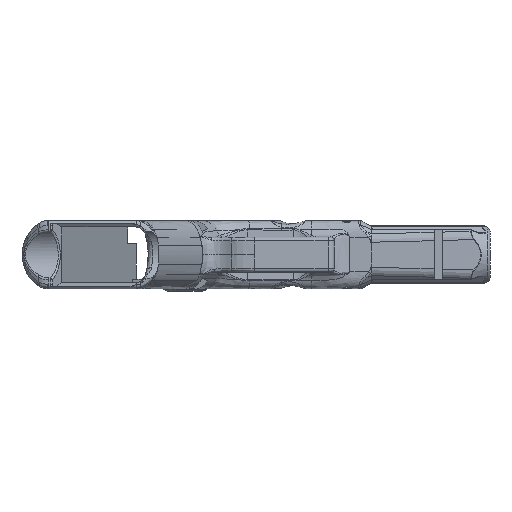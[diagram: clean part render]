
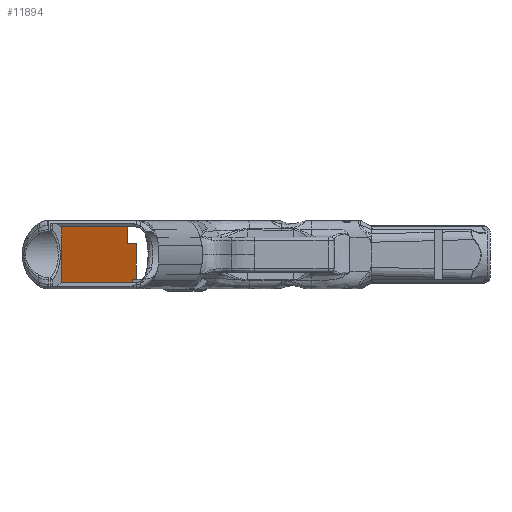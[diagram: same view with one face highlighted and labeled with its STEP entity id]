
A CAD part, front view. The second image highlights one B-rep face of the part: STEP entity #11894.
In plain terms, the highlighted planar face has unit normal (0.951, -0.309, 0).
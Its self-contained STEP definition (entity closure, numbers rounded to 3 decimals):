
#684=ELLIPSE('',#12474,1.051,1.);
#694=ELLIPSE('',#12501,1.051,1.);
#1610=FACE_OUTER_BOUND('',#2282,.T.);
#2282=EDGE_LOOP('',(#10482,#10483,#10484,#10485,#10486,#10487,#10488,#10489,
#10490,#10491));
#3350=LINE('',#25282,#4028);
#3474=LINE('',#29733,#4152);
#3485=LINE('',#30019,#4163);
#3627=LINE('',#42026,#4305);
#3650=LINE('',#43778,#4328);
#3654=LINE('',#44102,#4332);
#3660=LINE('',#44735,#4338);
#3661=LINE('',#44736,#4339);
#4028=VECTOR('',#13857,10.);
#4152=VECTOR('',#14323,10.);
#4163=VECTOR('',#14362,10.);
#4305=VECTOR('',#14990,10.);
#4328=VECTOR('',#15133,10.);
#4332=VECTOR('',#15141,10.);
#4338=VECTOR('',#15177,10.);
#4339=VECTOR('',#15178,10.);
#4899=VERTEX_POINT('',#25279);
#4900=VERTEX_POINT('',#25281);
#5053=VERTEX_POINT('',#28687);
#5094=VERTEX_POINT('',#29708);
#5096=VERTEX_POINT('',#29712);
#5104=VERTEX_POINT('',#29731);
#5458=VERTEX_POINT('',#42024);
#5495=VERTEX_POINT('',#43777);
#5502=VERTEX_POINT('',#44099);
#5503=VERTEX_POINT('',#44101);
#6274=EDGE_CURVE('',#4900,#4899,#3350,.T.);
#6515=EDGE_CURVE('',#5053,#4899,#684,.F.);
#6574=EDGE_CURVE('',#5096,#5094,#694,.F.);
#6584=EDGE_CURVE('',#5096,#5104,#3474,.T.);
#6614=EDGE_CURVE('',#5094,#5053,#3485,.F.);
#7158=EDGE_CURVE('',#5458,#5104,#3627,.T.);
#7235=EDGE_CURVE('',#5495,#5458,#3650,.T.);
#7245=EDGE_CURVE('',#5502,#5503,#3654,.T.);
#7262=EDGE_CURVE('',#5503,#5495,#3660,.T.);
#7263=EDGE_CURVE('',#4900,#5502,#3661,.T.);
#10482=ORIENTED_EDGE('',*,*,#6274,.T.);
#10483=ORIENTED_EDGE('',*,*,#6515,.F.);
#10484=ORIENTED_EDGE('',*,*,#6614,.F.);
#10485=ORIENTED_EDGE('',*,*,#6574,.F.);
#10486=ORIENTED_EDGE('',*,*,#6584,.T.);
#10487=ORIENTED_EDGE('',*,*,#7158,.F.);
#10488=ORIENTED_EDGE('',*,*,#7235,.F.);
#10489=ORIENTED_EDGE('',*,*,#7262,.F.);
#10490=ORIENTED_EDGE('',*,*,#7245,.F.);
#10491=ORIENTED_EDGE('',*,*,#7263,.F.);
#11324=PLANE('',#12836);
#11894=ADVANCED_FACE('',(#1610),#11324,.F.);
#12474=AXIS2_PLACEMENT_3D('',#28688,#14249,#14250);
#12501=AXIS2_PLACEMENT_3D('',#29714,#14310,#14311);
#12836=AXIS2_PLACEMENT_3D('',#44734,#15175,#15176);
#13857=DIRECTION('',(-0.309,-0.951,0.));
#14249=DIRECTION('center_axis',(-0.951,0.309,0.));
#14250=DIRECTION('ref_axis',(-0.309,-0.951,0.));
#14310=DIRECTION('center_axis',(-0.951,0.309,0.));
#14311=DIRECTION('ref_axis',(-0.309,-0.951,0.));
#14323=DIRECTION('',(0.309,0.951,0.));
#14362=DIRECTION('',(0.,0.,-1.));
#14990=DIRECTION('',(0.,0.,-1.));
#15133=DIRECTION('',(-0.309,-0.951,0.));
#15141=DIRECTION('',(0.309,0.951,0.));
#15175=DIRECTION('center_axis',(-0.951,0.309,0.));
#15176=DIRECTION('ref_axis',(0.,0.,
1.));
#15177=DIRECTION('',(0.,0.,-1.));
#15178=DIRECTION('',(0.,0.,-1.));
#25279=CARTESIAN_POINT('',(2.294,-97.822,11.75));
#25281=CARTESIAN_POINT('',(30.049,-12.4,11.75));
#25282=CARTESIAN_POINT('',(2.312,-97.765,11.75));
#28687=CARTESIAN_POINT('',(2.236,-98.,11.766));
#28688=CARTESIAN_POINT('Origin',(2.294,-97.822,12.75));
#29708=CARTESIAN_POINT('',(2.236,-98.,-11.766));
#29712=CARTESIAN_POINT('',(2.294,-97.822,-11.75));
#29714=CARTESIAN_POINT('Origin',(2.294,-97.822,-12.75));
#29731=CARTESIAN_POINT('',(32.169,-5.875,-11.75));
#29733=CARTESIAN_POINT('',(2.312,-97.765,-11.75));
#30019=CARTESIAN_POINT('',(2.236,-98.,-18.375));
#42024=CARTESIAN_POINT('',(32.169,-5.875,-10.375));
#42026=CARTESIAN_POINT('',(32.169,-5.875,-5.875));
#43777=CARTESIAN_POINT('',(33.591,-1.5,-10.375));
#43778=CARTESIAN_POINT('',(17.241,-51.82,-10.375));
#44099=CARTESIAN_POINT('',(30.049,-12.4,4.75));
#44101=CARTESIAN_POINT('',(33.591,-1.5,4.75));
#44102=CARTESIAN_POINT('',(18.86,-46.836,4.75));
#44734=CARTESIAN_POINT('Origin',(2.312,-97.765,-11.75));
#44735=CARTESIAN_POINT('',(33.591,-1.5,-5.875));
#44736=CARTESIAN_POINT('',(30.049,-12.4,2.982));
